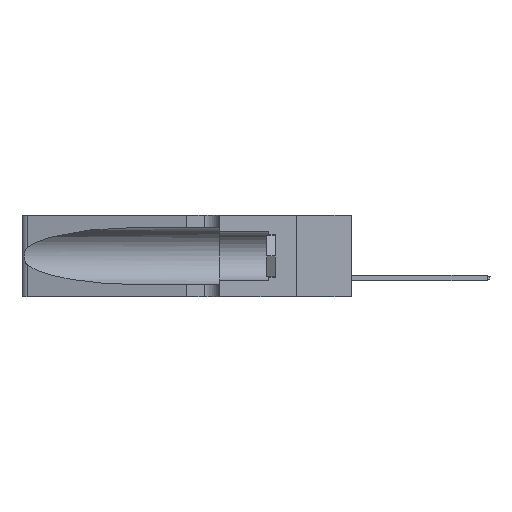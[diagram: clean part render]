
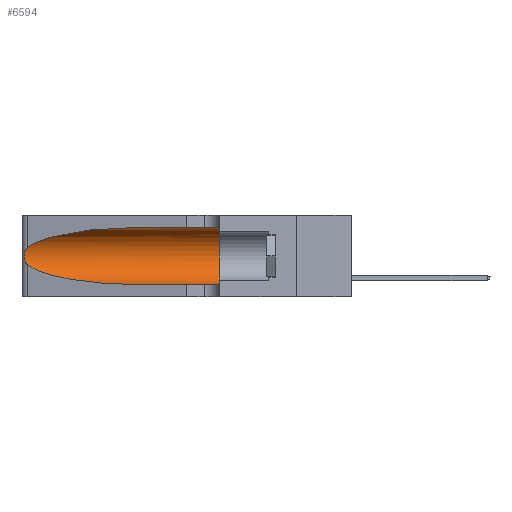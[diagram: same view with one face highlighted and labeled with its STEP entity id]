
A CAD part, left-side view. The second image highlights one B-rep face of the part: STEP entity #6594.
In plain terms, the highlighted cylindrical face has radius 3.308 mm (diameter 6.617 mm), a partial arc.
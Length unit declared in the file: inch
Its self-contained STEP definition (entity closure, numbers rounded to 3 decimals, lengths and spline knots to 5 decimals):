
#164 = ORIENTED_EDGE ( 'NONE', *, *, #4636, .T. ) ;
#831 = EDGE_CURVE ( 'NONE', #5338, #13928, #18265, .T. ) ;
#843 = CARTESIAN_POINT ( 'NONE',  ( 0.1305, 1.61858, 0.05475 ) ) ;
#1698 = DIRECTION ( 'NONE',  ( 0., -1., 0. ) ) ;
#2305 = CARTESIAN_POINT ( 'NONE',  ( 0.1305, 0.72297, 0.31525 ) ) ;
#2759 = ORIENTED_EDGE ( 'NONE', *, *, #12278, .T. ) ;
#3178 = EDGE_CURVE ( 'NONE', #15057, #17692, #18255, .T. ) ;
#3818 = CARTESIAN_POINT ( 'NONE',  ( 0.25555, 1.22994, 0.2215 ) ) ;
#4091 = CARTESIAN_POINT ( 'NONE',  ( 0.1305, 0.35, 0.31525 ) ) ;
#4335 = CARTESIAN_POINT ( 'NONE',  ( 0.25555, 1.22993, 0.14849 ) ) ;
#4504 = EDGE_LOOP ( 'NONE', ( #2759, #164, #6167, #23499, #6431, #28259 ) ) ;
#4636 = EDGE_CURVE ( 'NONE', #28458, #15057, #12094, .T. ) ;
#4789 = CARTESIAN_POINT ( 'NONE',  ( 0.1305, 0.35, 0.185 ) ) ;
#5054 = CIRCLE ( 'NONE', #31325, 0.13025 ) ;
#5338 = VERTEX_POINT ( 'NONE', #34903 ) ;
#6167 = ORIENTED_EDGE ( 'NONE', *, *, #3178, .T. ) ;
#6431 = ORIENTED_EDGE ( 'NONE', *, *, #19955, .F. ) ;
#6594 = ADVANCED_FACE ( 'NONE', ( #8044 ), #31438, .F. ) ;
#6917 = CARTESIAN_POINT ( 'NONE',  ( 0.25487, 1.22718, 0.22369 ) ) ;
#7342 = CARTESIAN_POINT ( 'NONE',  ( 0.26075, 1.23896, 0.19203 ) ) ;
#8044 = FACE_OUTER_BOUND ( 'NONE', #4504, .T. ) ;
#8169 = CARTESIAN_POINT ( 'NONE',  ( 0.25487, 1.22718, 0.14631 ) ) ;
#9738 = CARTESIAN_POINT ( 'NONE',  ( 0.25787, 1.23484, 0.2124 ) ) ;
#11551 = CARTESIAN_POINT ( 'NONE',  ( 0.25487, 1.22718, 0.14631 ) ) ;
#11750 = DIRECTION ( 'NONE',  ( 0., -1., 0. ) ) ;
#12094 = B_SPLINE_CURVE_WITH_KNOTS ( 'NONE', 3,
 ( #12826, #3818, #24444, #9738, #18761, #13514, #7342, #33767, #30943, #16464, #36621, #16210, #4335, #34041 ),
 .UNSPECIFIED., .F., .F.,
 ( 4, 2, 2, 2, 2, 2, 4 ),
 ( 0., 0.00027, 0.00053, 0.00107, 0.0016, 0.00187, 0.00214 ),
 .UNSPECIFIED. ) ;
#12278 = EDGE_CURVE ( 'NONE', #5338, #28458, #17369, .T. ) ;
#12826 = CARTESIAN_POINT ( 'NONE',  ( 0.25487, 1.22718, 0.22369 ) ) ;
#13514 = CARTESIAN_POINT ( 'NONE',  ( 0.26018, 1.23835, 0.19895 ) ) ;
#13928 = VERTEX_POINT ( 'NONE', #4091 ) ;
#15057 = VERTEX_POINT ( 'NONE', #8169 ) ;
#16210 = CARTESIAN_POINT ( 'NONE',  ( 0.25639, 1.23186, 0.15144 ) ) ;
#16257 = DIRECTION ( 'NONE',  ( 0., 0., 1. ) ) ;
#16464 = CARTESIAN_POINT ( 'NONE',  ( 0.25856, 1.23593, 0.16098 ) ) ;
#17369 =( BOUNDED_CURVE ( )  B_SPLINE_CURVE ( 3, ( #2305, #24825, #18748, #6917 ),
 .UNSPECIFIED., .F., .F. ) 
 B_SPLINE_CURVE_WITH_KNOTS ( ( 4, 4 ),
 ( 1.5708, 2.84003 ),
 .UNSPECIFIED. ) 
 CURVE ( )  GEOMETRIC_REPRESENTATION_ITEM ( )  RATIONAL_B_SPLINE_CURVE ( ( 1., 0.87, 0.87, 1. ) ) 
 REPRESENTATION_ITEM ( '' )  );
#17661 = EDGE_CURVE ( 'NONE', #17692, #25749, #28260, .T. ) ;
#17692 = VERTEX_POINT ( 'NONE', #30803 ) ;
#18255 =( BOUNDED_CURVE ( )  B_SPLINE_CURVE ( 3, ( #11551, #26013, #35207, #20597 ),
 .UNSPECIFIED., .F., .F. ) 
 B_SPLINE_CURVE_WITH_KNOTS ( ( 4, 4 ),
 ( 3.44316, 4.71239 ),
 .UNSPECIFIED. ) 
 CURVE ( )  GEOMETRIC_REPRESENTATION_ITEM ( )  RATIONAL_B_SPLINE_CURVE ( ( 1., 0.87, 0.87, 1. ) ) 
 REPRESENTATION_ITEM ( '' )  );
#18265 = LINE ( 'NONE', #25450, #37151 ) ;
#18748 = CARTESIAN_POINT ( 'NONE',  ( 0.2373, 1.15595, 0.28018 ) ) ;
#18761 = CARTESIAN_POINT ( 'NONE',  ( 0.25854, 1.2359, 0.20912 ) ) ;
#19437 = CARTESIAN_POINT ( 'NONE',  ( 0.1305, 0.35, 0.05475 ) ) ;
#19729 = DIRECTION ( 'NONE',  ( 0., 0., -1. ) ) ;
#19955 = EDGE_CURVE ( 'NONE', #13928, #25749, #5054, .T. ) ;
#20597 = CARTESIAN_POINT ( 'NONE',  ( 0.1305, 0.72297, 0.05475 ) ) ;
#20809 = AXIS2_PLACEMENT_3D ( 'NONE', #28421, #1698, #19729 ) ;
#21250 = CARTESIAN_POINT ( 'NONE',  ( 0.25487, 1.22718, 0.22369 ) ) ;
#23499 = ORIENTED_EDGE ( 'NONE', *, *, #17661, .T. ) ;
#24444 = CARTESIAN_POINT ( 'NONE',  ( 0.25639, 1.23184, 0.21858 ) ) ;
#24825 = CARTESIAN_POINT ( 'NONE',  ( 0.18966, 0.96281, 0.31525 ) ) ;
#25025 = DIRECTION ( 'NONE',  ( 0., 1., 0. ) ) ;
#25450 = CARTESIAN_POINT ( 'NONE',  ( 0.1305, 1.61858, 0.31525 ) ) ;
#25749 = VERTEX_POINT ( 'NONE', #19437 ) ;
#26013 = CARTESIAN_POINT ( 'NONE',  ( 0.2373, 1.15595, 0.08982 ) ) ;
#28259 = ORIENTED_EDGE ( 'NONE', *, *, #831, .F. ) ;
#28260 = LINE ( 'NONE', #843, #35163 ) ;
#28421 = CARTESIAN_POINT ( 'NONE',  ( 0.1305, 1.61858, 0.185 ) ) ;
#28458 = VERTEX_POINT ( 'NONE', #21250 ) ;
#30803 = CARTESIAN_POINT ( 'NONE',  ( 0.1305, 0.72297, 0.05475 ) ) ;
#30943 = CARTESIAN_POINT ( 'NONE',  ( 0.26017, 1.23833, 0.17102 ) ) ;
#31325 = AXIS2_PLACEMENT_3D ( 'NONE', #4789, #25025, #16257 ) ;
#31438 = CYLINDRICAL_SURFACE ( 'NONE', #20809, 0.13025 ) ;
#33222 = DIRECTION ( 'NONE',  ( 0., -1., 0. ) ) ;
#33767 = CARTESIAN_POINT ( 'NONE',  ( 0.26075, 1.23896, 0.178 ) ) ;
#34041 = CARTESIAN_POINT ( 'NONE',  ( 0.25487, 1.22718, 0.14631 ) ) ;
#34903 = CARTESIAN_POINT ( 'NONE',  ( 0.1305, 0.72297, 0.31525 ) ) ;
#35163 = VECTOR ( 'NONE', #33222, 39.37008 ) ;
#35207 = CARTESIAN_POINT ( 'NONE',  ( 0.18966, 0.96281, 0.05475 ) ) ;
#36621 = CARTESIAN_POINT ( 'NONE',  ( 0.25789, 1.23486, 0.15765 ) ) ;
#37151 = VECTOR ( 'NONE', #11750, 39.37008 ) ;
